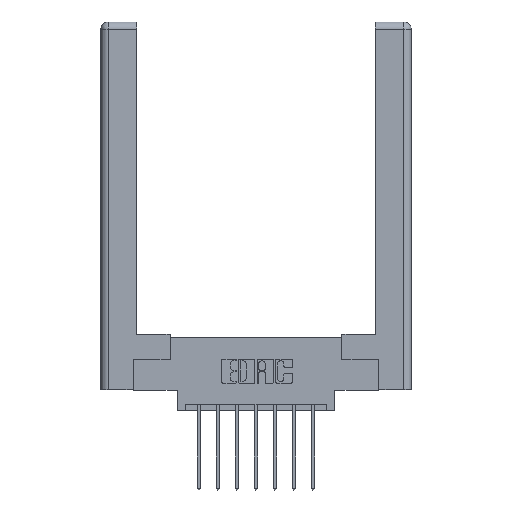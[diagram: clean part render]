
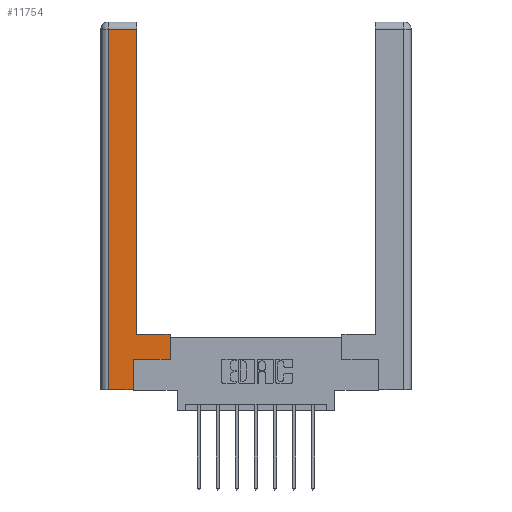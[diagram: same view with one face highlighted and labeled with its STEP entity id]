
A CAD part, top view. The second image highlights one B-rep face of the part: STEP entity #11754.
In plain terms, the highlighted planar face has unit normal (0, 0, 1).
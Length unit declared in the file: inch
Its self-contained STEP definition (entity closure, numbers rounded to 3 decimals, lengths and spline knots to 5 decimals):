
#102 = LINE ( 'NONE', #9868, #6695 ) ;
#366 = DIRECTION ( 'NONE',  ( 0., 0., -1. ) ) ;
#403 = ORIENTED_EDGE ( 'NONE', *, *, #3752, .T. ) ;
#476 = CARTESIAN_POINT ( 'NONE',  ( 0.565, 0.45, 0. ) ) ;
#900 = VERTEX_POINT ( 'NONE', #7162 ) ;
#1300 = VECTOR ( 'NONE', #9462, 39.37008 ) ;
#1336 = EDGE_CURVE ( 'NONE', #2601, #10539, #4142, .T. ) ;
#1552 = VECTOR ( 'NONE', #4542, 39.37008 ) ;
#1556 = VECTOR ( 'NONE', #7080, 39.37008 ) ;
#1558 = VECTOR ( 'NONE', #4143, 39.37008 ) ;
#2143 = CARTESIAN_POINT ( 'NONE',  ( 0.565, 0.245, 0. ) ) ;
#2157 = CARTESIAN_POINT ( 'NONE',  ( 0.565, 0.245, 0. ) ) ;
#2570 = EDGE_LOOP ( 'NONE', ( #8727, #3764, #9559, #2801, #9151, #9838, #4035, #403 ) ) ;
#2601 = VERTEX_POINT ( 'NONE', #9011 ) ;
#2623 = VERTEX_POINT ( 'NONE', #2143 ) ;
#2718 = LINE ( 'NONE', #5609, #6258 ) ;
#2801 = ORIENTED_EDGE ( 'NONE', *, *, #12150, .T. ) ;
#3049 = VECTOR ( 'NONE', #4916, 39.37008 ) ;
#3752 = EDGE_CURVE ( 'NONE', #10294, #7614, #10810, .T. ) ;
#3756 = CARTESIAN_POINT ( 'NONE',  ( 0.565, 0.45, 0. ) ) ;
#3764 = ORIENTED_EDGE ( 'NONE', *, *, #1336, .T. ) ;
#4035 = ORIENTED_EDGE ( 'NONE', *, *, #6181, .T. ) ;
#4142 = LINE ( 'NONE', #11375, #1552 ) ;
#4143 = DIRECTION ( 'NONE',  ( 0., -1., 0. ) ) ;
#4294 = LINE ( 'NONE', #12129, #1558 ) ;
#4542 = DIRECTION ( 'NONE',  ( -1., 0., 0. ) ) ;
#4730 = CARTESIAN_POINT ( 'NONE',  ( 0.265, 0., 0. ) ) ;
#4744 = EDGE_CURVE ( 'NONE', #7614, #2601, #2718, .T. ) ;
#4916 = DIRECTION ( 'NONE',  ( -1., 0., 0. ) ) ;
#4922 = VERTEX_POINT ( 'NONE', #10147 ) ;
#5609 = CARTESIAN_POINT ( 'NONE',  ( 0.295, 3., 0. ) ) ;
#5655 = VECTOR ( 'NONE', #10788, 39.37008 ) ;
#6181 = EDGE_CURVE ( 'NONE', #2623, #10294, #6862, .T. ) ;
#6258 = VECTOR ( 'NONE', #7683, 39.37008 ) ;
#6264 = CARTESIAN_POINT ( 'NONE',  ( 0., 0., 0. ) ) ;
#6695 = VECTOR ( 'NONE', #8901, 39.37008 ) ;
#6720 = EDGE_CURVE ( 'NONE', #4922, #900, #102, .T. ) ;
#6862 = LINE ( 'NONE', #476, #1300 ) ;
#7080 = DIRECTION ( 'NONE',  ( 1., 0., 0. ) ) ;
#7162 = CARTESIAN_POINT ( 'NONE',  ( 0.265, 0.245, 0. ) ) ;
#7248 = DIRECTION ( 'NONE',  ( -1., 0., 0. ) ) ;
#7614 = VERTEX_POINT ( 'NONE', #11731 ) ;
#7683 = DIRECTION ( 'NONE',  ( 0., 1., 0. ) ) ;
#8131 = CARTESIAN_POINT ( 'NONE',  ( 0.295, 0.45, 0. ) ) ;
#8511 = CARTESIAN_POINT ( 'NONE',  ( 0.0615, 0., 0. ) ) ;
#8626 = FACE_OUTER_BOUND ( 'NONE', #2570, .T. ) ;
#8727 = ORIENTED_EDGE ( 'NONE', *, *, #4744, .T. ) ;
#8828 = EDGE_CURVE ( 'NONE', #10539, #8863, #4294, .T. ) ;
#8863 = VERTEX_POINT ( 'NONE', #8511 ) ;
#8901 = DIRECTION ( 'NONE',  ( 0., 1., 0. ) ) ;
#8962 = LINE ( 'NONE', #2157, #1556 ) ;
#9007 = PLANE ( 'NONE',  #11605 ) ;
#9011 = CARTESIAN_POINT ( 'NONE',  ( 0.295, 2.94, 0. ) ) ;
#9151 = ORIENTED_EDGE ( 'NONE', *, *, #6720, .T. ) ;
#9436 = EDGE_CURVE ( 'NONE', #900, #2623, #8962, .T. ) ;
#9462 = DIRECTION ( 'NONE',  ( 0., 1., 0. ) ) ;
#9559 = ORIENTED_EDGE ( 'NONE', *, *, #8828, .T. ) ;
#9838 = ORIENTED_EDGE ( 'NONE', *, *, #9436, .T. ) ;
#9868 = CARTESIAN_POINT ( 'NONE',  ( 0.265, 0.245, 0. ) ) ;
#10147 = CARTESIAN_POINT ( 'NONE',  ( 0.265, 0., 0. ) ) ;
#10158 = LINE ( 'NONE', #4730, #5655 ) ;
#10294 = VERTEX_POINT ( 'NONE', #3756 ) ;
#10539 = VERTEX_POINT ( 'NONE', #10648 ) ;
#10648 = CARTESIAN_POINT ( 'NONE',  ( 0.0615, 2.94, 0. ) ) ;
#10788 = DIRECTION ( 'NONE',  ( 1., 0., 0. ) ) ;
#10810 = LINE ( 'NONE', #8131, #3049 ) ;
#11375 = CARTESIAN_POINT ( 'NONE',  ( 0.0615, 2.94, 0. ) ) ;
#11605 = AXIS2_PLACEMENT_3D ( 'NONE', #6264, #366, #7248 ) ;
#11731 = CARTESIAN_POINT ( 'NONE',  ( 0.295, 0.45, 0. ) ) ;
#11754 = ADVANCED_FACE ( 'NONE', ( #8626 ), #9007, .F. ) ;
#12129 = CARTESIAN_POINT ( 'NONE',  ( 0.0615, 0., 0. ) ) ;
#12150 = EDGE_CURVE ( 'NONE', #8863, #4922, #10158, .T. ) ;
